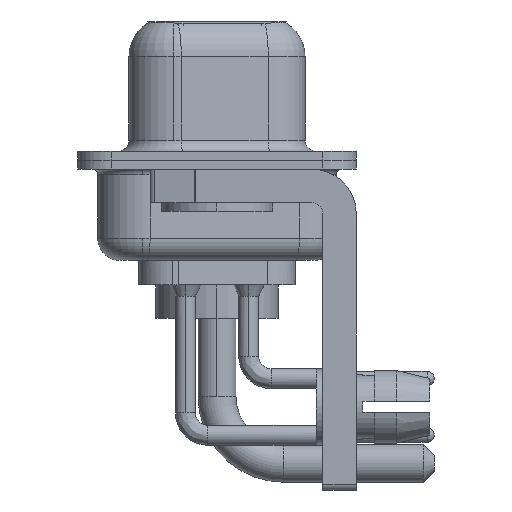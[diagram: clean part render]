
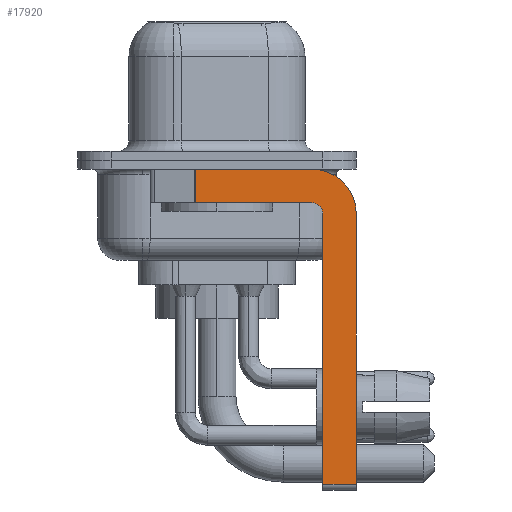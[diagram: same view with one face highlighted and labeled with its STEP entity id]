
A CAD part, left-side view. The second image highlights one B-rep face of the part: STEP entity #17920.
In plain terms, the highlighted planar face has unit normal (-1, 0, 0).
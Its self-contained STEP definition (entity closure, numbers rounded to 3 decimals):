
#45 = EDGE_CURVE ( 'NONE', #11946, #11153, #18616, .T. ) ;
#110 = EDGE_CURVE ( 'NONE', #11153, #1049, #4864, .T. ) ;
#164 = ORIENTED_EDGE ( 'NONE', *, *, #110, .F. ) ;
#701 = VECTOR ( 'NONE', #9726, 1000. ) ;
#831 = AXIS2_PLACEMENT_3D ( 'NONE', #18014, #2508, #1077 ) ;
#853 = CARTESIAN_POINT ( 'NONE',  ( -2.9, -4.25, -0.4 ) ) ;
#1049 = VERTEX_POINT ( 'NONE', #6545 ) ;
#1077 = DIRECTION ( 'NONE',  ( 0., 0., 1. ) ) ;
#2508 = DIRECTION ( 'NONE',  ( -1., 0., 0. ) ) ;
#2656 = CIRCLE ( 'NONE', #831, 0.5 ) ;
#2695 = CARTESIAN_POINT ( 'NONE',  ( -2.9, -4.75, -2.4 ) ) ;
#3080 = DIRECTION ( 'NONE',  ( 0., 1., 0. ) ) ;
#3528 = ORIENTED_EDGE ( 'NONE', *, *, #45, .F. ) ;
#3631 = DIRECTION ( 'NONE',  ( 0., 0., -1. ) ) ;
#4383 = DIRECTION ( 'NONE',  ( 0., 0., -1. ) ) ;
#4864 = LINE ( 'NONE', #12241, #6841 ) ;
#4989 = LINE ( 'NONE', #12276, #701 ) ;
#5071 = VECTOR ( 'NONE', #7107, 1000. ) ;
#5137 = CARTESIAN_POINT ( 'NONE',  ( -2.9, -4.25, -2.4 ) ) ;
#5207 = CARTESIAN_POINT ( 'NONE',  ( -2.9, -4.75, -14.8 ) ) ;
#5798 = PLANE ( 'NONE',  #6098 ) ;
#5895 = CARTESIAN_POINT ( 'NONE',  ( -2.9, -4.25, -2.4 ) ) ;
#6098 = AXIS2_PLACEMENT_3D ( 'NONE', #5895, #11673, #4383 ) ;
#6214 = EDGE_CURVE ( 'NONE', #13708, #17377, #8226, .T. ) ;
#6503 = CARTESIAN_POINT ( 'NONE',  ( -2.9, -4.25, -14.55 ) ) ;
#6545 = CARTESIAN_POINT ( 'NONE',  ( -2.9, -6.25, -14.55 ) ) ;
#6563 = EDGE_CURVE ( 'NONE', #8314, #13708, #2656, .T. ) ;
#6841 = VECTOR ( 'NONE', #3631, 1000. ) ;
#7107 = DIRECTION ( 'NONE',  ( 0., 0., -1. ) ) ;
#7386 = CARTESIAN_POINT ( 'NONE',  ( -2.9, -4.25, -1.9 ) ) ;
#7429 = CARTESIAN_POINT ( 'NONE',  ( -2.9, -4.25, -1.9 ) ) ;
#7897 = DIRECTION ( 'NONE',  ( 0., 0., -1. ) ) ;
#8212 = ORIENTED_EDGE ( 'NONE', *, *, #9516, .T. ) ;
#8226 = LINE ( 'NONE', #7429, #8436 ) ;
#8314 = VERTEX_POINT ( 'NONE', #2695 ) ;
#8436 = VECTOR ( 'NONE', #3080, 1000. ) ;
#8747 = FACE_OUTER_BOUND ( 'NONE', #8983, .T. ) ;
#8983 = EDGE_LOOP ( 'NONE', ( #9421, #14609, #17381, #17804, #17995, #8212, #164, #3528 ) ) ;
#9186 = VERTEX_POINT ( 'NONE', #11932 ) ;
#9362 = LINE ( 'NONE', #6503, #13008 ) ;
#9421 = ORIENTED_EDGE ( 'NONE', *, *, #18501, .F. ) ;
#9516 = EDGE_CURVE ( 'NONE', #9186, #1049, #9362, .T. ) ;
#9663 = LINE ( 'NONE', #5207, #15706 ) ;
#9726 = DIRECTION ( 'NONE',  ( 0., -1., 0. ) ) ;
#9842 = CARTESIAN_POINT ( 'NONE',  ( -2.9, 0.978, -0.4 ) ) ;
#10055 = LINE ( 'NONE', #15829, #5071 ) ;
#11093 = AXIS2_PLACEMENT_3D ( 'NONE', #5137, #16414, #7897 ) ;
#11153 = VERTEX_POINT ( 'NONE', #15690 ) ;
#11673 = DIRECTION ( 'NONE',  ( 1., 0., 0. ) ) ;
#11932 = CARTESIAN_POINT ( 'NONE',  ( -2.9, -4.75, -14.55 ) ) ;
#11946 = VERTEX_POINT ( 'NONE', #853 ) ;
#12241 = CARTESIAN_POINT ( 'NONE',  ( -2.9, -6.25, -2.4 ) ) ;
#12276 = CARTESIAN_POINT ( 'NONE',  ( -2.9, 3., -0.4 ) ) ;
#13008 = VECTOR ( 'NONE', #17676, 1000. ) ;
#13477 = CARTESIAN_POINT ( 'NONE',  ( -2.9, 0.978, -1.9 ) ) ;
#13653 = EDGE_CURVE ( 'NONE', #14025, #17377, #10055, .T. ) ;
#13708 = VERTEX_POINT ( 'NONE', #7386 ) ;
#14025 = VERTEX_POINT ( 'NONE', #9842 ) ;
#14609 = ORIENTED_EDGE ( 'NONE', *, *, #13653, .T. ) ;
#15200 = EDGE_CURVE ( 'NONE', #9186, #8314, #9663, .T. ) ;
#15690 = CARTESIAN_POINT ( 'NONE',  ( -2.9, -6.25, -2.4 ) ) ;
#15706 = VECTOR ( 'NONE', #16571, 1000. ) ;
#15829 = CARTESIAN_POINT ( 'NONE',  ( -2.9, 0.978, -1.9 ) ) ;
#16414 = DIRECTION ( 'NONE',  ( 1., 0., 0. ) ) ;
#16571 = DIRECTION ( 'NONE',  ( 0., 0., 1. ) ) ;
#17377 = VERTEX_POINT ( 'NONE', #13477 ) ;
#17381 = ORIENTED_EDGE ( 'NONE', *, *, #6214, .F. ) ;
#17676 = DIRECTION ( 'NONE',  ( 0., -1., 0. ) ) ;
#17804 = ORIENTED_EDGE ( 'NONE', *, *, #6563, .F. ) ;
#17920 = ADVANCED_FACE ( 'NONE', ( #8747 ), #5798, .F. ) ;
#17995 = ORIENTED_EDGE ( 'NONE', *, *, #15200, .F. ) ;
#18014 = CARTESIAN_POINT ( 'NONE',  ( -2.9, -4.25, -2.4 ) ) ;
#18501 = EDGE_CURVE ( 'NONE', #14025, #11946, #4989, .T. ) ;
#18616 = CIRCLE ( 'NONE', #11093, 2. ) ;
